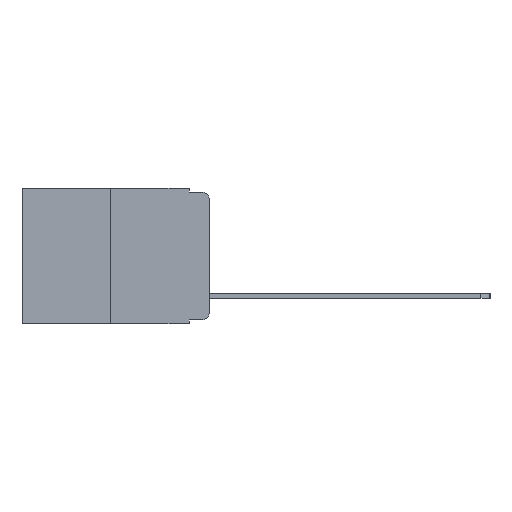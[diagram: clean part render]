
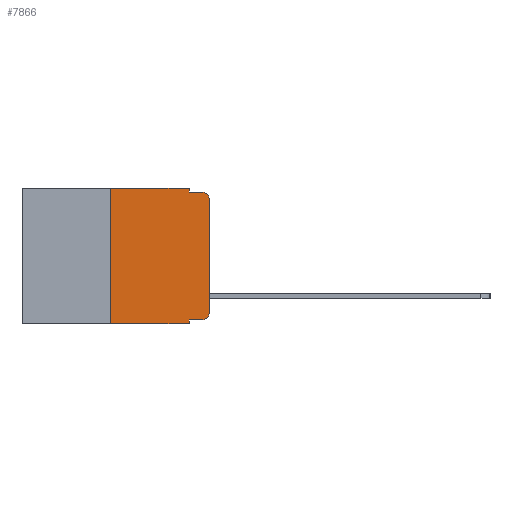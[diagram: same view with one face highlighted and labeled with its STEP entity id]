
A CAD part, left-side view. The second image highlights one B-rep face of the part: STEP entity #7866.
In plain terms, the highlighted planar face has unit normal (-1, 0, 0).
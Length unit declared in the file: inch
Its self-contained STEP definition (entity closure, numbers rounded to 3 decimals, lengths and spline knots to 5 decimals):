
#71 = CARTESIAN_POINT ( 'NONE',  ( 0., 0.473, 0. ) ) ;
#160 = EDGE_CURVE ( 'NONE', #1465, #963, #20456, .T. ) ;
#597 = CARTESIAN_POINT ( 'NONE',  ( 0., 0.051, -0.01 ) ) ;
#963 = VERTEX_POINT ( 'NONE', #21270 ) ;
#1285 = DIRECTION ( 'NONE',  ( 0., 0., -1. ) ) ;
#1465 = VERTEX_POINT ( 'NONE', #7817 ) ;
#1805 = DIRECTION ( 'NONE',  ( 1., 0., 0. ) ) ;
#1982 = CARTESIAN_POINT ( 'NONE',  ( 0., 0.25, 0. ) ) ;
#2111 = CARTESIAN_POINT ( 'NONE',  ( 0., 0.473, -0.343 ) ) ;
#2370 = EDGE_CURVE ( 'NONE', #8540, #4717, #10166, .T. ) ;
#2589 = LINE ( 'NONE', #6447, #9965 ) ;
#2749 = CARTESIAN_POINT ( 'NONE',  ( 0., 0.051, -0.343 ) ) ;
#3221 = ORIENTED_EDGE ( 'NONE', *, *, #13627, .T. ) ;
#3664 = AXIS2_PLACEMENT_3D ( 'NONE', #71, #1805, #13517 ) ;
#4028 = VECTOR ( 'NONE', #8175, 39.37008 ) ;
#4029 = CIRCLE ( 'NONE', #21046, 0.02 ) ;
#4134 = DIRECTION ( 'NONE',  ( 0., 0., -1. ) ) ;
#4297 = LINE ( 'NONE', #7533, #8289 ) ;
#4436 = LINE ( 'NONE', #9695, #11019 ) ;
#4550 = LINE ( 'NONE', #18048, #4028 ) ;
#4644 = ORIENTED_EDGE ( 'NONE', *, *, #20433, .T. ) ;
#4688 = ORIENTED_EDGE ( 'NONE', *, *, #17186, .F. ) ;
#4717 = VERTEX_POINT ( 'NONE', #2749 ) ;
#4722 = DIRECTION ( 'NONE',  ( 0., -1., 0. ) ) ;
#4850 = VERTEX_POINT ( 'NONE', #19607 ) ;
#5219 = AXIS2_PLACEMENT_3D ( 'NONE', #19367, #9560, #21001 ) ;
#5922 = EDGE_CURVE ( 'NONE', #8540, #9783, #17692, .T. ) ;
#6175 = ORIENTED_EDGE ( 'NONE', *, *, #10041, .F. ) ;
#6220 = ORIENTED_EDGE ( 'NONE', *, *, #13850, .F. ) ;
#6447 = CARTESIAN_POINT ( 'NONE',  ( 0., 0.051, -0.333 ) ) ;
#6737 = CARTESIAN_POINT ( 'NONE',  ( 0., 0.051, 0. ) ) ;
#7063 = CARTESIAN_POINT ( 'NONE',  ( 0., 0.02, -0.01 ) ) ;
#7533 = CARTESIAN_POINT ( 'NONE',  ( 0., 0., 0. ) ) ;
#7817 = CARTESIAN_POINT ( 'NONE',  ( 0., 0.02, -0.333 ) ) ;
#7866 = ADVANCED_FACE ( 'NONE', ( #20540 ), #19974, .F. ) ;
#8175 = DIRECTION ( 'NONE',  ( 0., -1., 0. ) ) ;
#8289 = VECTOR ( 'NONE', #14212, 39.37008 ) ;
#8540 = VERTEX_POINT ( 'NONE', #15520 ) ;
#9560 = DIRECTION ( 'NONE',  ( -1., 0., 0. ) ) ;
#9695 = CARTESIAN_POINT ( 'NONE',  ( 0., 0.051, -0.01 ) ) ;
#9783 = VERTEX_POINT ( 'NONE', #1982 ) ;
#9965 = VECTOR ( 'NONE', #4722, 39.37008 ) ;
#10041 = EDGE_CURVE ( 'NONE', #4850, #10777, #15918, .T. ) ;
#10166 = LINE ( 'NONE', #2111, #13532 ) ;
#10777 = VERTEX_POINT ( 'NONE', #597 ) ;
#10886 = CARTESIAN_POINT ( 'NONE',  ( 0., 0.051, 0. ) ) ;
#11019 = VECTOR ( 'NONE', #11379, 39.37008 ) ;
#11198 = ORIENTED_EDGE ( 'NONE', *, *, #5922, .F. ) ;
#11333 = VERTEX_POINT ( 'NONE', #7063 ) ;
#11379 = DIRECTION ( 'NONE',  ( 0., -1., 0. ) ) ;
#11388 = DIRECTION ( 'NONE',  ( -1., 0., 0. ) ) ;
#11682 = ORIENTED_EDGE ( 'NONE', *, *, #2370, .T. ) ;
#11863 = EDGE_LOOP ( 'NONE', ( #3221, #4644, #4688, #6175, #6220, #11198, #11682, #17590, #17608, #18131 ) ) ;
#12187 = DIRECTION ( 'NONE',  ( 0., -1., 0. ) ) ;
#12711 = VECTOR ( 'NONE', #4134, 39.37008 ) ;
#13234 = CARTESIAN_POINT ( 'NONE',  ( 0., 0.25, 0. ) ) ;
#13517 = DIRECTION ( 'NONE',  ( 0., 0., -1. ) ) ;
#13532 = VECTOR ( 'NONE', #12187, 39.37008 ) ;
#13627 = EDGE_CURVE ( 'NONE', #963, #14433, #4297, .T. ) ;
#13850 = EDGE_CURVE ( 'NONE', #9783, #4850, #4550, .T. ) ;
#14212 = DIRECTION ( 'NONE',  ( 0., 0., 1. ) ) ;
#14332 = CARTESIAN_POINT ( 'NONE',  ( 0., 0.051, -0.333 ) ) ;
#14433 = VERTEX_POINT ( 'NONE', #15693 ) ;
#14472 = EDGE_CURVE ( 'NONE', #18267, #4717, #21365, .T. ) ;
#14870 = DIRECTION ( 'NONE',  ( 0., 0., 1. ) ) ;
#14898 = VECTOR ( 'NONE', #14870, 39.37008 ) ;
#15408 = VECTOR ( 'NONE', #19931, 39.37008 ) ;
#15520 = CARTESIAN_POINT ( 'NONE',  ( 0., 0.25, -0.343 ) ) ;
#15693 = CARTESIAN_POINT ( 'NONE',  ( 0., 0., -0.03 ) ) ;
#15918 = LINE ( 'NONE', #6737, #15408 ) ;
#17186 = EDGE_CURVE ( 'NONE', #10777, #11333, #4436, .T. ) ;
#17590 = ORIENTED_EDGE ( 'NONE', *, *, #14472, .F. ) ;
#17608 = ORIENTED_EDGE ( 'NONE', *, *, #18421, .T. ) ;
#17692 = LINE ( 'NONE', #13234, #14898 ) ;
#18048 = CARTESIAN_POINT ( 'NONE',  ( 0., 0.473, 0. ) ) ;
#18131 = ORIENTED_EDGE ( 'NONE', *, *, #160, .T. ) ;
#18267 = VERTEX_POINT ( 'NONE', #14332 ) ;
#18421 = EDGE_CURVE ( 'NONE', #18267, #1465, #2589, .T. ) ;
#19367 = CARTESIAN_POINT ( 'NONE',  ( 0., 0.02, -0.313 ) ) ;
#19607 = CARTESIAN_POINT ( 'NONE',  ( 0., 0.051, 0. ) ) ;
#19931 = DIRECTION ( 'NONE',  ( 0., 0., -1. ) ) ;
#19974 = PLANE ( 'NONE',  #3664 ) ;
#20433 = EDGE_CURVE ( 'NONE', #14433, #11333, #4029, .T. ) ;
#20456 = CIRCLE ( 'NONE', #5219, 0.02 ) ;
#20540 = FACE_OUTER_BOUND ( 'NONE', #11863, .T. ) ;
#21001 = DIRECTION ( 'NONE',  ( 0., 0., -1. ) ) ;
#21046 = AXIS2_PLACEMENT_3D ( 'NONE', #21142, #11388, #1285 ) ;
#21142 = CARTESIAN_POINT ( 'NONE',  ( 0., 0.02, -0.03 ) ) ;
#21270 = CARTESIAN_POINT ( 'NONE',  ( 0., 0., -0.313 ) ) ;
#21365 = LINE ( 'NONE', #10886, #12711 ) ;
